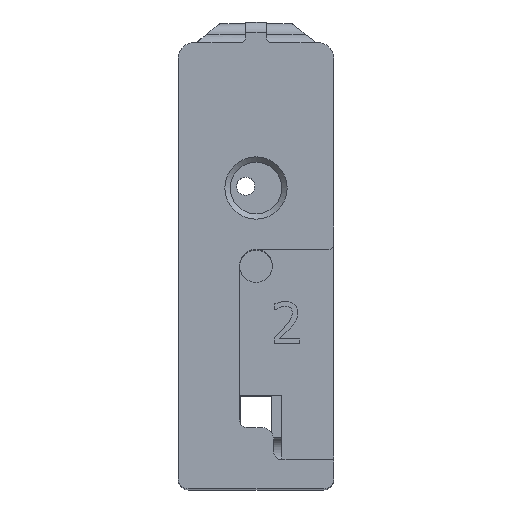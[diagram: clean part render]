
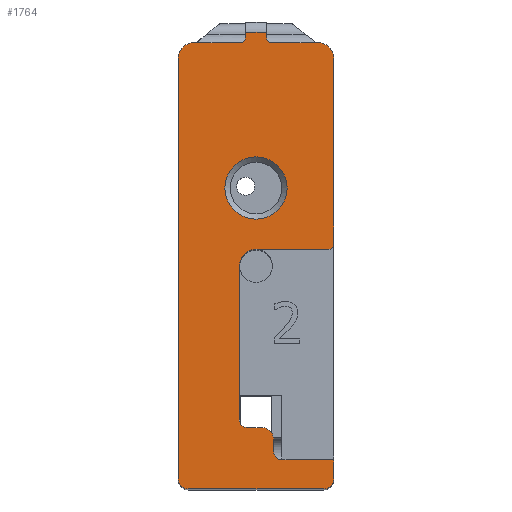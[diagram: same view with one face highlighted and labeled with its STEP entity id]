
A CAD part, top view. The second image highlights one B-rep face of the part: STEP entity #1764.
In plain terms, the highlighted planar face has unit normal (0, 0, 1).
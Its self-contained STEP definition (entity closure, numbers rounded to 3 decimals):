
#1402=CARTESIAN_POINT('',(5.,-37.4,16.));
#1403=VERTEX_POINT('',#1402);
#1410=CARTESIAN_POINT('',(15.0,-37.4,16.));
#1411=VERTEX_POINT('',#1410);
#1412=CARTESIAN_POINT('',(15.,-37.4,16.));
#1413=DIRECTION('',(-1.0,0.0,0.0));
#1414=VECTOR('',#1413,10.);
#1415=LINE('',#1412,#1414);
#1416=EDGE_CURVE('',#1411,#1403,#1415,.T.);
#1434=CARTESIAN_POINT('',(-3.2,-29.6,16.));
#1435=VERTEX_POINT('',#1434);
#1442=CARTESIAN_POINT('',(-1.6,-31.2,16.));
#1443=VERTEX_POINT('',#1442);
#1444=CARTESIAN_POINT('',(-1.6,-29.6,16.));
#1445=DIRECTION('',(0.0,0.0,1.0));
#1446=DIRECTION('',(-0.707,-0.707,0.0));
#1447=AXIS2_PLACEMENT_3D('',#1444,#1445,#1446);
#1448=CIRCLE('',#1447,1.6);
#1449=EDGE_CURVE('',#1435,#1443,#1448,.T.);
#1467=CARTESIAN_POINT('',(-3.2,0.0,16.));
#1468=VERTEX_POINT('',#1467);
#1475=CARTESIAN_POINT('',(-3.2,-29.6,16.));
#1476=DIRECTION('',(0.0,1.0,0.0));
#1477=VECTOR('',#1476,29.6);
#1478=LINE('',#1475,#1477);
#1479=EDGE_CURVE('',#1435,#1468,#1478,.T.);
#1493=CARTESIAN_POINT('',(3.4,-35.8,16.));
#1494=VERTEX_POINT('',#1493);
#1501=CARTESIAN_POINT('',(5.,-35.8,16.));
#1502=DIRECTION('',(0.0,0.0,1.0));
#1503=DIRECTION('',(-0.707,-0.707,0.0));
#1504=AXIS2_PLACEMENT_3D('',#1501,#1502,#1503);
#1505=CIRCLE('',#1504,1.6);
#1506=EDGE_CURVE('',#1494,#1403,#1505,.T.);
#1520=CARTESIAN_POINT('',(3.4,-33.4,16.));
#1521=VERTEX_POINT('',#1520);
#1528=CARTESIAN_POINT('',(3.4,-35.8,16.));
#1529=DIRECTION('',(0.0,1.0,0.0));
#1530=VECTOR('',#1529,2.4);
#1531=LINE('',#1528,#1530);
#1532=EDGE_CURVE('',#1494,#1521,#1531,.T.);
#1542=CARTESIAN_POINT('',(15.0,4.2,16.));
#1543=VERTEX_POINT('',#1542);
#1544=CARTESIAN_POINT('',(14.0,3.2,16.));
#1545=VERTEX_POINT('',#1544);
#1546=CARTESIAN_POINT('',(14.0,4.2,16.));
#1547=DIRECTION('',(0.0,0.0,-1.0));
#1548=DIRECTION('',(0.707,-0.707,0.0));
#1549=AXIS2_PLACEMENT_3D('',#1546,#1547,#1548);
#1550=CIRCLE('',#1549,1.0);
#1551=EDGE_CURVE('',#1543,#1545,#1550,.T.);
#1575=CARTESIAN_POINT('',(0.0,3.2,16.));
#1576=VERTEX_POINT('',#1575);
#1577=CARTESIAN_POINT('',(0.0,3.2,16.));
#1578=DIRECTION('',(1.0,0.0,0.0));
#1579=VECTOR('',#1578,14.0);
#1580=LINE('',#1577,#1579);
#1581=EDGE_CURVE('',#1576,#1545,#1580,.T.);
#1593=CARTESIAN_POINT('',(0.0,0.,16.));
#1594=DIRECTION('',(0.0,0.0,1.0));
#1595=DIRECTION('',(1.0,0.0,0.0));
#1596=AXIS2_PLACEMENT_3D('',#1593,#1594,#1595);
#1597=PLANE('',#1596);
#1598=ORIENTED_EDGE('',*,*,#1551,.F.);
#1599=CARTESIAN_POINT('',(15.0,40.,16.));
#1600=VERTEX_POINT('',#1599);
#1601=CARTESIAN_POINT('',(15.0,4.2,16.));
#1602=DIRECTION('',(0.0,1.0,0.0));
#1603=VECTOR('',#1602,35.8);
#1604=LINE('',#1601,#1603);
#1605=EDGE_CURVE('',#1543,#1600,#1604,.T.);
#1606=ORIENTED_EDGE('',*,*,#1605,.T.);
#1607=CARTESIAN_POINT('',(12.0,43.,16.));
#1608=VERTEX_POINT('',#1607);
#1609=CARTESIAN_POINT('',(12.0,40.,16.));
#1610=DIRECTION('',(0.0,0.0,-1.0));
#1611=DIRECTION('',(0.707,0.707,0.0));
#1612=AXIS2_PLACEMENT_3D('',#1609,#1610,#1611);
#1613=CIRCLE('',#1612,3.0);
#1614=EDGE_CURVE('',#1608,#1600,#1613,.T.);
#1615=ORIENTED_EDGE('',*,*,#1614,.F.);
#1616=CARTESIAN_POINT('',(3.0,43.,16.));
#1617=VERTEX_POINT('',#1616);
#1618=CARTESIAN_POINT('',(3.0,43.,16.));
#1619=DIRECTION('',(1.0,0.0,0.0));
#1620=VECTOR('',#1619,9.0);
#1621=LINE('',#1618,#1620);
#1622=EDGE_CURVE('',#1617,#1608,#1621,.T.);
#1623=ORIENTED_EDGE('',*,*,#1622,.F.);
#1624=CARTESIAN_POINT('',(2.0,44.,16.));
#1625=VERTEX_POINT('',#1624);
#1626=CARTESIAN_POINT('',(3.0,44.,16.));
#1627=DIRECTION('',(0.0,0.0,1.0));
#1628=DIRECTION('',(-0.707,-0.707,0.0));
#1629=AXIS2_PLACEMENT_3D('',#1626,#1627,#1628);
#1630=CIRCLE('',#1629,1.0);
#1631=EDGE_CURVE('',#1625,#1617,#1630,.T.);
#1632=ORIENTED_EDGE('',*,*,#1631,.F.);
#1633=CARTESIAN_POINT('',(2.0,45.,16.));
#1634=VERTEX_POINT('',#1633);
#1635=CARTESIAN_POINT('',(2.0,44.,16.));
#1636=DIRECTION('',(0.0,1.0,0.0));
#1637=VECTOR('',#1636,1.);
#1638=LINE('',#1635,#1637);
#1639=EDGE_CURVE('',#1625,#1634,#1638,.T.);
#1640=ORIENTED_EDGE('',*,*,#1639,.T.);
#1641=CARTESIAN_POINT('',(-2.0,45.,16.));
#1642=VERTEX_POINT('',#1641);
#1643=CARTESIAN_POINT('',(-2.0,45.,16.));
#1644=DIRECTION('',(1.0,0.0,0.0));
#1645=VECTOR('',#1644,4.0);
#1646=LINE('',#1643,#1645);
#1647=EDGE_CURVE('',#1642,#1634,#1646,.T.);
#1648=ORIENTED_EDGE('',*,*,#1647,.F.);
#1649=CARTESIAN_POINT('',(-2.0,44.,16.));
#1650=VERTEX_POINT('',#1649);
#1651=CARTESIAN_POINT('',(-2.0,45.,16.));
#1652=DIRECTION('',(0.0,-1.0,0.0));
#1653=VECTOR('',#1652,1.);
#1654=LINE('',#1651,#1653);
#1655=EDGE_CURVE('',#1642,#1650,#1654,.T.);
#1656=ORIENTED_EDGE('',*,*,#1655,.T.);
#1657=CARTESIAN_POINT('',(-3.0,43.,16.));
#1658=VERTEX_POINT('',#1657);
#1659=CARTESIAN_POINT('',(-3.0,44.,16.));
#1660=DIRECTION('',(0.0,0.0,1.0));
#1661=DIRECTION('',(0.707,-0.707,0.0));
#1662=AXIS2_PLACEMENT_3D('',#1659,#1660,#1661);
#1663=CIRCLE('',#1662,1.0);
#1664=EDGE_CURVE('',#1658,#1650,#1663,.T.);
#1665=ORIENTED_EDGE('',*,*,#1664,.F.);
#1666=CARTESIAN_POINT('',(-12.0,43.,16.));
#1667=VERTEX_POINT('',#1666);
#1668=CARTESIAN_POINT('',(-12.0,43.,16.));
#1669=DIRECTION('',(1.0,0.0,0.0));
#1670=VECTOR('',#1669,9.0);
#1671=LINE('',#1668,#1670);
#1672=EDGE_CURVE('',#1667,#1658,#1671,.T.);
#1673=ORIENTED_EDGE('',*,*,#1672,.F.);
#1674=CARTESIAN_POINT('',(-15.0,40.,16.));
#1675=VERTEX_POINT('',#1674);
#1676=CARTESIAN_POINT('',(-12.0,40.,16.));
#1677=DIRECTION('',(0.0,0.0,-1.0));
#1678=DIRECTION('',(-0.707,0.707,0.0));
#1679=AXIS2_PLACEMENT_3D('',#1676,#1677,#1678);
#1680=CIRCLE('',#1679,3.0);
#1681=EDGE_CURVE('',#1675,#1667,#1680,.T.);
#1682=ORIENTED_EDGE('',*,*,#1681,.F.);
#1683=CARTESIAN_POINT('',(-15.0,-41.,16.));
#1684=VERTEX_POINT('',#1683);
#1685=CARTESIAN_POINT('',(-15.0,40.,16.));
#1686=DIRECTION('',(0.0,-1.0,0.0));
#1687=VECTOR('',#1686,81.);
#1688=LINE('',#1685,#1687);
#1689=EDGE_CURVE('',#1675,#1684,#1688,.T.);
#1690=ORIENTED_EDGE('',*,*,#1689,.T.);
#1691=CARTESIAN_POINT('',(-13.0,-43.,16.));
#1692=VERTEX_POINT('',#1691);
#1693=CARTESIAN_POINT('',(-13.0,-41.,16.));
#1694=DIRECTION('',(0.0,0.0,-1.0));
#1695=DIRECTION('',(-0.707,-0.707,0.0));
#1696=AXIS2_PLACEMENT_3D('',#1693,#1694,#1695);
#1697=CIRCLE('',#1696,2.0);
#1698=EDGE_CURVE('',#1692,#1684,#1697,.T.);
#1699=ORIENTED_EDGE('',*,*,#1698,.F.);
#1700=CARTESIAN_POINT('',(13.0,-43.,16.));
#1701=VERTEX_POINT('',#1700);
#1702=CARTESIAN_POINT('',(-13.0,-43.,16.));
#1703=DIRECTION('',(1.0,0.0,0.0));
#1704=VECTOR('',#1703,26.0);
#1705=LINE('',#1702,#1704);
#1706=EDGE_CURVE('',#1692,#1701,#1705,.T.);
#1707=ORIENTED_EDGE('',*,*,#1706,.T.);
#1708=CARTESIAN_POINT('',(15.0,-41.,16.));
#1709=VERTEX_POINT('',#1708);
#1710=CARTESIAN_POINT('',(13.0,-41.,16.));
#1711=DIRECTION('',(0.0,0.0,-1.0));
#1712=DIRECTION('',(0.707,-0.707,0.0));
#1713=AXIS2_PLACEMENT_3D('',#1710,#1711,#1712);
#1714=CIRCLE('',#1713,2.0);
#1715=EDGE_CURVE('',#1709,#1701,#1714,.T.);
#1716=ORIENTED_EDGE('',*,*,#1715,.F.);
#1717=CARTESIAN_POINT('',(15.0,-41.,16.));
#1718=DIRECTION('',(0.0,1.0,0.0));
#1719=VECTOR('',#1718,3.6);
#1720=LINE('',#1717,#1719);
#1721=EDGE_CURVE('',#1709,#1411,#1720,.T.);
#1722=ORIENTED_EDGE('',*,*,#1721,.T.);
#1723=ORIENTED_EDGE('',*,*,#1416,.T.);
#1724=ORIENTED_EDGE('',*,*,#1506,.F.);
#1725=ORIENTED_EDGE('',*,*,#1532,.T.);
#1726=CARTESIAN_POINT('',(1.2,-31.2,16.));
#1727=VERTEX_POINT('',#1726);
#1728=CARTESIAN_POINT('',(1.2,-33.4,16.));
#1729=DIRECTION('',(0.0,0.0,-1.0));
#1730=DIRECTION('',(0.707,0.707,0.0));
#1731=AXIS2_PLACEMENT_3D('',#1728,#1729,#1730);
#1732=CIRCLE('',#1731,2.2);
#1733=EDGE_CURVE('',#1727,#1521,#1732,.T.);
#1734=ORIENTED_EDGE('',*,*,#1733,.F.);
#1735=CARTESIAN_POINT('',(1.2,-31.2,16.));
#1736=DIRECTION('',(-1.0,0.0,0.0));
#1737=VECTOR('',#1736,2.8);
#1738=LINE('',#1735,#1737);
#1739=EDGE_CURVE('',#1727,#1443,#1738,.T.);
#1740=ORIENTED_EDGE('',*,*,#1739,.T.);
#1741=ORIENTED_EDGE('',*,*,#1449,.F.);
#1742=ORIENTED_EDGE('',*,*,#1479,.T.);
#1743=CARTESIAN_POINT('',(0.0,0.0,16.));
#1744=DIRECTION('',(0.0,0.0,-1.0));
#1745=DIRECTION('',(-1.0,0.0,0.0));
#1746=AXIS2_PLACEMENT_3D('',#1743,#1744,#1745);
#1747=CIRCLE('',#1746,3.2);
#1748=EDGE_CURVE('',#1468,#1576,#1747,.T.);
#1749=ORIENTED_EDGE('',*,*,#1748,.T.);
#1750=ORIENTED_EDGE('',*,*,#1581,.T.);
#1751=EDGE_LOOP('',(#1598,#1606,#1615,#1623,#1632,#1640,#1648,#1656,#1665,#1673,#1682,#1690,#1699,#1707,#1716,#1722,#1723,#1724,#1725,#1734,#1740,#1741,#1742,#1749,#1750));
#1752=FACE_OUTER_BOUND('',#1751,.T.);
#1753=CARTESIAN_POINT('',(6.0,15.0,16.));
#1754=VERTEX_POINT('',#1753);
#1755=CARTESIAN_POINT('',(0.0,15.0,16.));
#1756=DIRECTION('',(0.0,0.0,1.0));
#1757=DIRECTION('',(-1.0,0.0,0.0));
#1758=AXIS2_PLACEMENT_3D('',#1755,#1756,#1757);
#1759=CIRCLE('',#1758,6.0);
#1760=EDGE_CURVE('',#1754,#1754,#1759,.T.);
#1761=ORIENTED_EDGE('',*,*,#1760,.F.);
#1762=EDGE_LOOP('',(#1761));
#1763=FACE_BOUND('',#1762,.T.);
#1764=ADVANCED_FACE('',(#1752,#1763),#1597,.T.);
